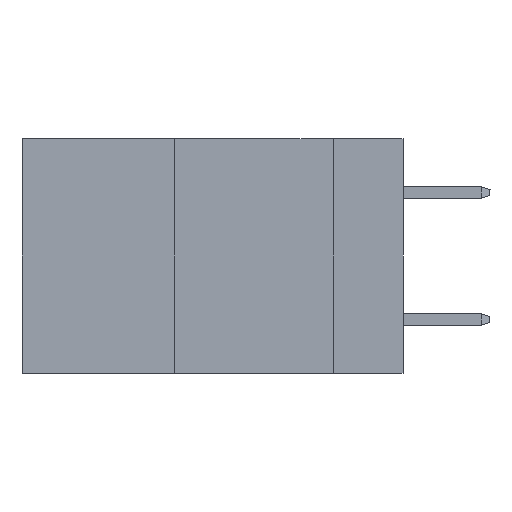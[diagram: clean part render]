
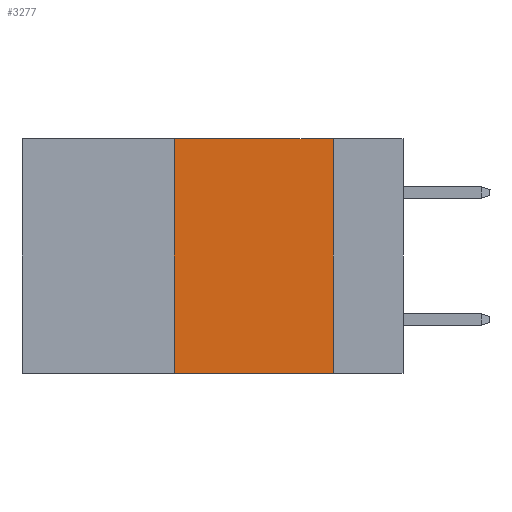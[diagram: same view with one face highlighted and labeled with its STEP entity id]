
A CAD part, left-side view. The second image highlights one B-rep face of the part: STEP entity #3277.
In plain terms, the highlighted planar face has unit normal (-1, 0, 0).
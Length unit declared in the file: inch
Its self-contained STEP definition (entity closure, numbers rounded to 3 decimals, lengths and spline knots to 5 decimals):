
#5 = DIRECTION ( 'NONE',  ( 0., 0., -1. ) ) ;
#233 = CARTESIAN_POINT ( 'NONE',  ( 0., 0.11, -0.37 ) ) ;
#1121 = VERTEX_POINT ( 'NONE', #5394 ) ;
#1478 = EDGE_CURVE ( 'NONE', #11133, #7973, #20786, .T. ) ;
#3168 = CARTESIAN_POINT ( 'NONE',  ( 0., 0.11, 0. ) ) ;
#3277 = ADVANCED_FACE ( 'NONE', ( #15610 ), #10641, .F. ) ;
#4205 = DIRECTION ( 'NONE',  ( 0., -1., 0. ) ) ;
#4315 = ORIENTED_EDGE ( 'NONE', *, *, #7451, .F. ) ;
#5394 = CARTESIAN_POINT ( 'NONE',  ( 0., 0.36, -0.37 ) ) ;
#5699 = CARTESIAN_POINT ( 'NONE',  ( 0., 0.6, 0. ) ) ;
#7002 = CARTESIAN_POINT ( 'NONE',  ( 0., 0.36, 0. ) ) ;
#7451 = EDGE_CURVE ( 'NONE', #1121, #11133, #20183, .T. ) ;
#7973 = VERTEX_POINT ( 'NONE', #3168 ) ;
#8794 = ORIENTED_EDGE ( 'NONE', *, *, #15035, .F. ) ;
#9788 = LINE ( 'NONE', #20781, #15519 ) ;
#9793 = DIRECTION ( 'NONE',  ( 0., -1., 0. ) ) ;
#9862 = VECTOR ( 'NONE', #19867, 39.37008 ) ;
#10539 = DIRECTION ( 'NONE',  ( 0., 0., -1. ) ) ;
#10641 = PLANE ( 'NONE',  #18497 ) ;
#10904 = CARTESIAN_POINT ( 'NONE',  ( 0., 0.6, -0.37 ) ) ;
#11133 = VERTEX_POINT ( 'NONE', #13878 ) ;
#11594 = VECTOR ( 'NONE', #4205, 39.37008 ) ;
#12195 = LINE ( 'NONE', #10904, #11594 ) ;
#12763 = CARTESIAN_POINT ( 'NONE',  ( 0., 0.6, 0. ) ) ;
#13621 = VERTEX_POINT ( 'NONE', #233 ) ;
#13878 = CARTESIAN_POINT ( 'NONE',  ( 0., 0.36, 0. ) ) ;
#15035 = EDGE_CURVE ( 'NONE', #7973, #13621, #9788, .T. ) ;
#15361 = VECTOR ( 'NONE', #9793, 39.37008 ) ;
#15519 = VECTOR ( 'NONE', #5, 39.37008 ) ;
#15610 = FACE_OUTER_BOUND ( 'NONE', #18682, .T. ) ;
#15879 = ORIENTED_EDGE ( 'NONE', *, *, #1478, .F. ) ;
#17086 = DIRECTION ( 'NONE',  ( 1., 0., 0. ) ) ;
#18497 = AXIS2_PLACEMENT_3D ( 'NONE', #5699, #17086, #10539 ) ;
#18682 = EDGE_LOOP ( 'NONE', ( #8794, #15879, #4315, #20804 ) ) ;
#19867 = DIRECTION ( 'NONE',  ( 0., 0., 1. ) ) ;
#20183 = LINE ( 'NONE', #7002, #9862 ) ;
#20781 = CARTESIAN_POINT ( 'NONE',  ( 0., 0.11, 0. ) ) ;
#20786 = LINE ( 'NONE', #12763, #15361 ) ;
#20803 = EDGE_CURVE ( 'NONE', #1121, #13621, #12195, .T. ) ;
#20804 = ORIENTED_EDGE ( 'NONE', *, *, #20803, .T. ) ;
